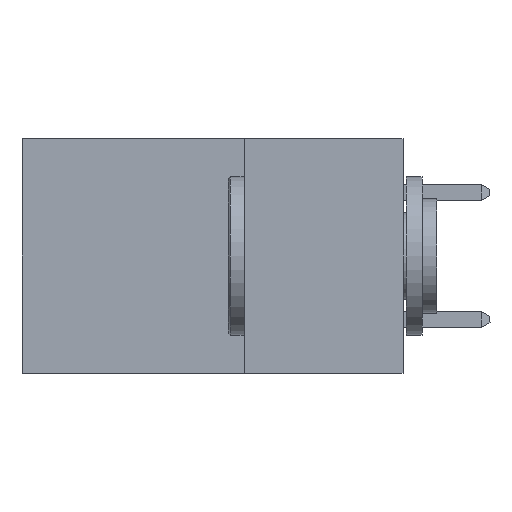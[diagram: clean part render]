
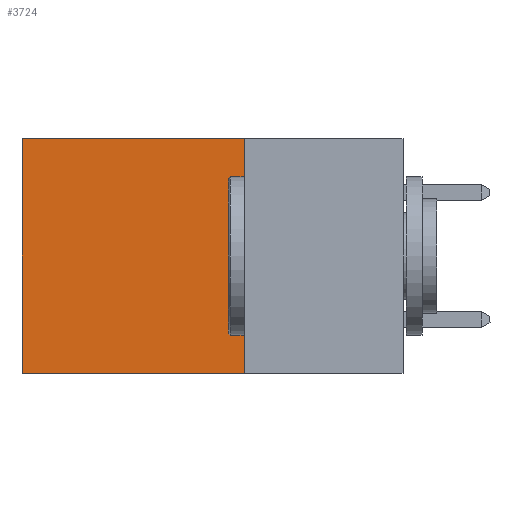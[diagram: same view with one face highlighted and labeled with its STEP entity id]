
A CAD part, left-side view. The second image highlights one B-rep face of the part: STEP entity #3724.
In plain terms, the highlighted planar face has unit normal (-1, 0, 0).
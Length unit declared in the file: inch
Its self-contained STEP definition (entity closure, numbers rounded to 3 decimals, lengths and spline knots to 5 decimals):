
#149 = ORIENTED_EDGE ( 'NONE', *, *, #2639, .F. ) ;
#178 = CARTESIAN_POINT ( 'NONE',  ( 0.2875, 0.25, 0. ) ) ;
#408 = DIRECTION ( 'NONE',  ( 0., 0., -1. ) ) ;
#567 = DIRECTION ( 'NONE',  ( 1., 0., 0. ) ) ;
#739 = PLANE ( 'NONE',  #1485 ) ;
#1008 = EDGE_CURVE ( 'NONE', #8928, #5887, #8977, .T. ) ;
#1374 = ORIENTED_EDGE ( 'NONE', *, *, #1008, .F. ) ;
#1485 = AXIS2_PLACEMENT_3D ( 'NONE', #1628, #567, #408 ) ;
#1489 = ORIENTED_EDGE ( 'NONE', *, *, #3056, .T. ) ;
#1628 = CARTESIAN_POINT ( 'NONE',  ( 0.2875, 0.25, 0. ) ) ;
#1683 = LINE ( 'NONE', #3891, #7597 ) ;
#1957 = VERTEX_POINT ( 'NONE', #9147 ) ;
#2623 = EDGE_CURVE ( 'NONE', #5972, #1957, #6041, .T. ) ;
#2639 = EDGE_CURVE ( 'NONE', #5887, #1957, #1683, .T. ) ;
#2660 = VECTOR ( 'NONE', #3576, 39.37008 ) ;
#2904 = CARTESIAN_POINT ( 'NONE',  ( 0.2875, 0.6, 0. ) ) ;
#2912 = LINE ( 'NONE', #3651, #2660 ) ;
#3014 = ORIENTED_EDGE ( 'NONE', *, *, #2623, .T. ) ;
#3056 = EDGE_CURVE ( 'NONE', #8928, #5972, #2912, .T. ) ;
#3576 = DIRECTION ( 'NONE',  ( 0., 1., 0. ) ) ;
#3617 = CARTESIAN_POINT ( 'NONE',  ( 0.2875, 0.25, 0. ) ) ;
#3651 = CARTESIAN_POINT ( 'NONE',  ( 0.2875, 0.25, 0. ) ) ;
#3724 = ADVANCED_FACE ( 'NONE', ( #7594 ), #739, .F. ) ;
#3797 = DIRECTION ( 'NONE',  ( 0., 0., -1. ) ) ;
#3891 = CARTESIAN_POINT ( 'NONE',  ( 0.2875, 0.25, -0.37 ) ) ;
#3904 = DIRECTION ( 'NONE',  ( 0., 1., 0. ) ) ;
#4558 = EDGE_LOOP ( 'NONE', ( #3014, #149, #1374, #1489 ) ) ;
#5887 = VERTEX_POINT ( 'NONE', #6824 ) ;
#5972 = VERTEX_POINT ( 'NONE', #7561 ) ;
#6041 = LINE ( 'NONE', #2904, #9240 ) ;
#6824 = CARTESIAN_POINT ( 'NONE',  ( 0.2875, 0.25, -0.37 ) ) ;
#6926 = DIRECTION ( 'NONE',  ( 0., 0., -1. ) ) ;
#7116 = VECTOR ( 'NONE', #6926, 39.37008 ) ;
#7561 = CARTESIAN_POINT ( 'NONE',  ( 0.2875, 0.6, 0. ) ) ;
#7594 = FACE_OUTER_BOUND ( 'NONE', #4558, .T. ) ;
#7597 = VECTOR ( 'NONE', #3904, 39.37008 ) ;
#8928 = VERTEX_POINT ( 'NONE', #178 ) ;
#8977 = LINE ( 'NONE', #3617, #7116 ) ;
#9147 = CARTESIAN_POINT ( 'NONE',  ( 0.2875, 0.6, -0.37 ) ) ;
#9240 = VECTOR ( 'NONE', #3797, 39.37008 ) ;
